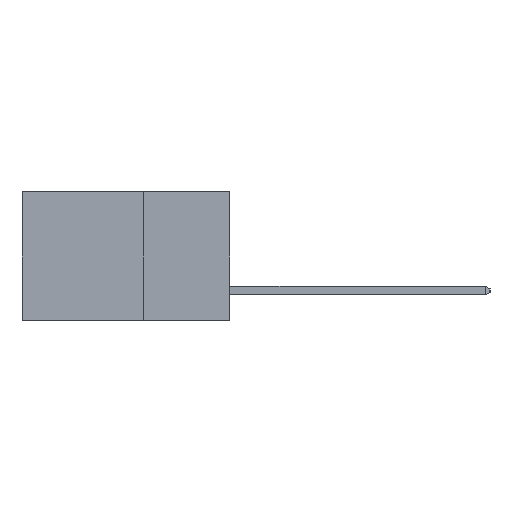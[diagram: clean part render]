
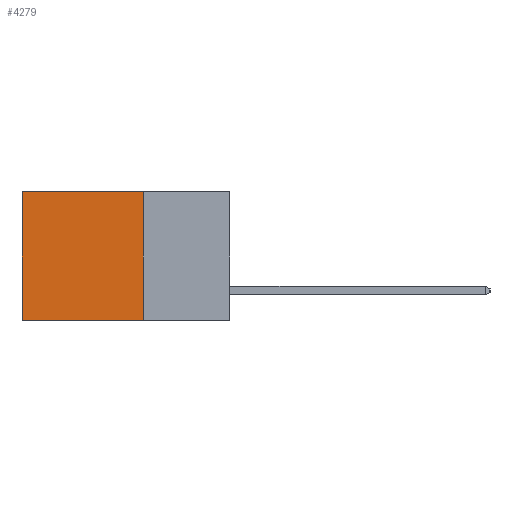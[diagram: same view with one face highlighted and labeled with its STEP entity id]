
A CAD part, left-side view. The second image highlights one B-rep face of the part: STEP entity #4279.
In plain terms, the highlighted planar face has unit normal (-1, 0, 0).
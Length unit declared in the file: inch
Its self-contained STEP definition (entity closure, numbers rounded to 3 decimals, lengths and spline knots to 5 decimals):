
#102 = VECTOR ( 'NONE', #2978, 39.37008 ) ;
#808 = FACE_OUTER_BOUND ( 'NONE', #12773, .T. ) ;
#1267 = CARTESIAN_POINT ( 'NONE',  ( 0.2615, 0.25, -0.37 ) ) ;
#1290 = DIRECTION ( 'NONE',  ( 0., 0., -1. ) ) ;
#1454 = CARTESIAN_POINT ( 'NONE',  ( 0.2615, 0.6, -0.37 ) ) ;
#1515 = VERTEX_POINT ( 'NONE', #8567 ) ;
#1869 = EDGE_CURVE ( 'NONE', #13559, #6103, #15551, .T. ) ;
#2327 = ORIENTED_EDGE ( 'NONE', *, *, #11848, .F. ) ;
#2332 = CARTESIAN_POINT ( 'NONE',  ( 0.2615, 0.25, -0.37 ) ) ;
#2806 = VERTEX_POINT ( 'NONE', #6342 ) ;
#2978 = DIRECTION ( 'NONE',  ( 0., 0., -1. ) ) ;
#3344 = CARTESIAN_POINT ( 'NONE',  ( 0.2615, 0.6, 0. ) ) ;
#3948 = DIRECTION ( 'NONE',  ( 0., 1., 0. ) ) ;
#4279 = ADVANCED_FACE ( 'NONE', ( #808 ), #11932, .F. ) ;
#5402 = DIRECTION ( 'NONE',  ( 0., 1., 0. ) ) ;
#6103 = VERTEX_POINT ( 'NONE', #3344 ) ;
#6342 = CARTESIAN_POINT ( 'NONE',  ( 0.2615, 0.6, -0.37 ) ) ;
#6755 = ORIENTED_EDGE ( 'NONE', *, *, #12412, .T. ) ;
#7373 = LINE ( 'NONE', #1267, #13862 ) ;
#7415 = CARTESIAN_POINT ( 'NONE',  ( 0.2615, 0.25, 0. ) ) ;
#7589 = VECTOR ( 'NONE', #5402, 39.37008 ) ;
#8050 = LINE ( 'NONE', #2332, #7589 ) ;
#8077 = CARTESIAN_POINT ( 'NONE',  ( 0.2615, 0.25, 0. ) ) ;
#8567 = CARTESIAN_POINT ( 'NONE',  ( 0.2615, 0.25, -0.37 ) ) ;
#9467 = AXIS2_PLACEMENT_3D ( 'NONE', #11195, #11255, #11130 ) ;
#11130 = DIRECTION ( 'NONE',  ( 0., 0., -1. ) ) ;
#11195 = CARTESIAN_POINT ( 'NONE',  ( 0.2615, 0.25, -0.37 ) ) ;
#11255 = DIRECTION ( 'NONE',  ( 1., 0., 0. ) ) ;
#11293 = LINE ( 'NONE', #1454, #102 ) ;
#11848 = EDGE_CURVE ( 'NONE', #13559, #1515, #7373, .T. ) ;
#11932 = PLANE ( 'NONE',  #9467 ) ;
#11967 = VECTOR ( 'NONE', #3948, 39.37008 ) ;
#12074 = ORIENTED_EDGE ( 'NONE', *, *, #17060, .F. ) ;
#12412 = EDGE_CURVE ( 'NONE', #6103, #2806, #11293, .T. ) ;
#12773 = EDGE_LOOP ( 'NONE', ( #6755, #12074, #2327, #14582 ) ) ;
#13559 = VERTEX_POINT ( 'NONE', #7415 ) ;
#13862 = VECTOR ( 'NONE', #1290, 39.37008 ) ;
#14582 = ORIENTED_EDGE ( 'NONE', *, *, #1869, .T. ) ;
#15551 = LINE ( 'NONE', #8077, #11967 ) ;
#17060 = EDGE_CURVE ( 'NONE', #1515, #2806, #8050, .T. ) ;
